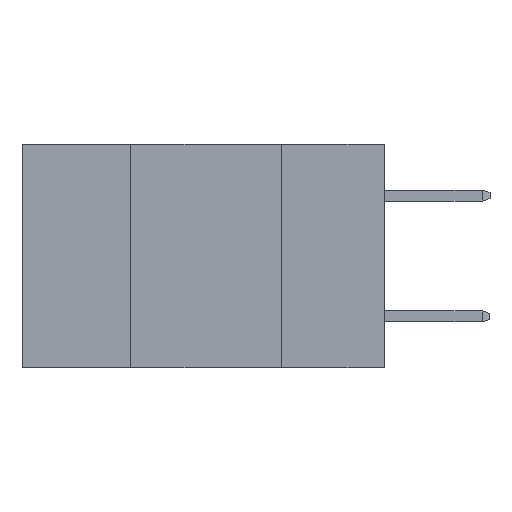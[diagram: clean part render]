
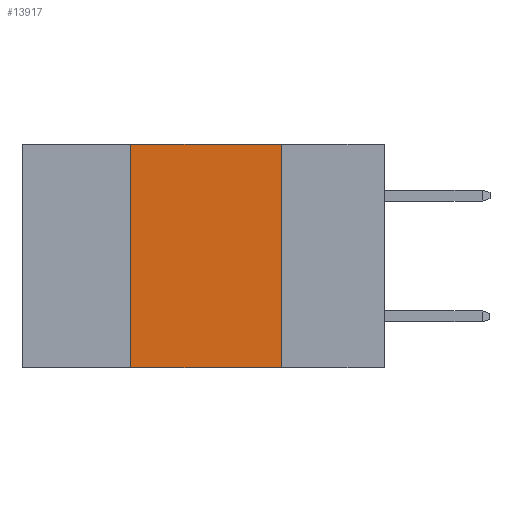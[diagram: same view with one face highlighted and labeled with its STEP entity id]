
A CAD part, left-side view. The second image highlights one B-rep face of the part: STEP entity #13917.
In plain terms, the highlighted planar face has unit normal (-1, 0, 0).
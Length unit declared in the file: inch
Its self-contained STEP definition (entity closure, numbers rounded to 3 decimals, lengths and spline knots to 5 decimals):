
#28 = EDGE_CURVE ( 'NONE', #15706, #14550, #9878, .T. ) ;
#167 = ORIENTED_EDGE ( 'NONE', *, *, #6717, .F. ) ;
#178 = CARTESIAN_POINT ( 'NONE',  ( 0., 0.17, -0.37 ) ) ;
#215 = DIRECTION ( 'NONE',  ( 0., 0., -1. ) ) ;
#986 = CARTESIAN_POINT ( 'NONE',  ( 0., 0.17, 0. ) ) ;
#1142 = PLANE ( 'NONE',  #16707 ) ;
#1340 = VECTOR ( 'NONE', #20043, 39.37008 ) ;
#2278 = VERTEX_POINT ( 'NONE', #178 ) ;
#2339 = VECTOR ( 'NONE', #215, 39.37008 ) ;
#2731 = CARTESIAN_POINT ( 'NONE',  ( 0., 0.6, 0. ) ) ;
#3205 = CARTESIAN_POINT ( 'NONE',  ( 0., 0.42, 0. ) ) ;
#4945 = ORIENTED_EDGE ( 'NONE', *, *, #28, .F. ) ;
#5368 = VERTEX_POINT ( 'NONE', #9580 ) ;
#5974 = DIRECTION ( 'NONE',  ( 0., 0., -1. ) ) ;
#6262 = DIRECTION ( 'NONE',  ( 0., 0., 1. ) ) ;
#6450 = CARTESIAN_POINT ( 'NONE',  ( 0., 0.42, 0. ) ) ;
#6717 = EDGE_CURVE ( 'NONE', #14550, #2278, #10840, .T. ) ;
#7971 = ORIENTED_EDGE ( 'NONE', *, *, #12921, .T. ) ;
#8109 = CARTESIAN_POINT ( 'NONE',  ( 0., 0.6, -0.37 ) ) ;
#8177 = EDGE_CURVE ( 'NONE', #5368, #15706, #9093, .T. ) ;
#9093 = LINE ( 'NONE', #6450, #16398 ) ;
#9580 = CARTESIAN_POINT ( 'NONE',  ( 0., 0.42, -0.37 ) ) ;
#9878 = LINE ( 'NONE', #20368, #1340 ) ;
#9880 = VECTOR ( 'NONE', #17470, 39.37008 ) ;
#10840 = LINE ( 'NONE', #986, #2339 ) ;
#12921 = EDGE_CURVE ( 'NONE', #5368, #2278, #18580, .T. ) ;
#13917 = ADVANCED_FACE ( 'NONE', ( #19068 ), #1142, .F. ) ;
#14307 = EDGE_LOOP ( 'NONE', ( #167, #4945, #15316, #7971 ) ) ;
#14550 = VERTEX_POINT ( 'NONE', #16294 ) ;
#15316 = ORIENTED_EDGE ( 'NONE', *, *, #8177, .F. ) ;
#15397 = DIRECTION ( 'NONE',  ( 1., 0., 0. ) ) ;
#15706 = VERTEX_POINT ( 'NONE', #3205 ) ;
#16294 = CARTESIAN_POINT ( 'NONE',  ( 0., 0.17, 0. ) ) ;
#16398 = VECTOR ( 'NONE', #6262, 39.37008 ) ;
#16707 = AXIS2_PLACEMENT_3D ( 'NONE', #2731, #15397, #5974 ) ;
#17470 = DIRECTION ( 'NONE',  ( 0., -1., 0. ) ) ;
#18580 = LINE ( 'NONE', #8109, #9880 ) ;
#19068 = FACE_OUTER_BOUND ( 'NONE', #14307, .T. ) ;
#20043 = DIRECTION ( 'NONE',  ( 0., -1., 0. ) ) ;
#20368 = CARTESIAN_POINT ( 'NONE',  ( 0., 0.6, 0. ) ) ;
